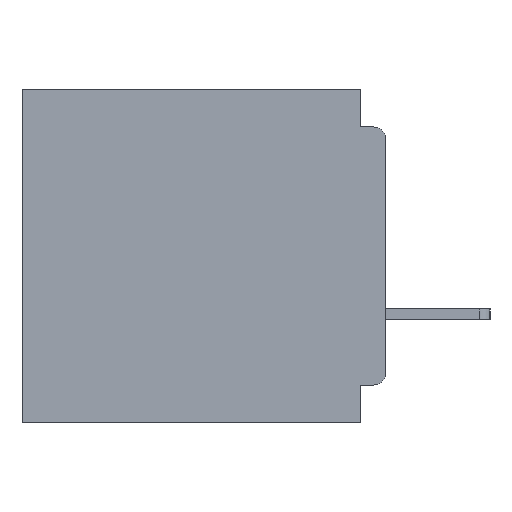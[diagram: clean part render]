
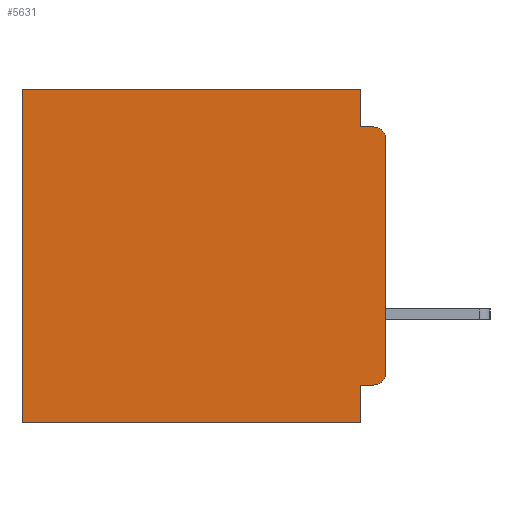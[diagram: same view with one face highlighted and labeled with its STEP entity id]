
A CAD part, left-side view. The second image highlights one B-rep face of the part: STEP entity #5631.
In plain terms, the highlighted planar face has unit normal (-1, 0, 0).
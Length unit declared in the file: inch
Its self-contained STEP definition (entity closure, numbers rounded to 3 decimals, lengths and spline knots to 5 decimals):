
#741 = EDGE_CURVE ( 'NONE', #38805, #25974, #11885, .T. ) ;
#1370 = DIRECTION ( 'NONE',  ( 0., 1., 0. ) ) ;
#1485 = CARTESIAN_POINT ( 'NONE',  ( 0.3, 0.031, -0.4 ) ) ;
#1677 = DIRECTION ( 'NONE',  ( 0., 0., -1. ) ) ;
#1824 = ORIENTED_EDGE ( 'NONE', *, *, #9214, .F. ) ;
#2013 = EDGE_CURVE ( 'NONE', #36168, #10395, #43363, .T. ) ;
#3082 = ORIENTED_EDGE ( 'NONE', *, *, #47708, .F. ) ;
#3362 = CARTESIAN_POINT ( 'NONE',  ( 0.3, 0.437, -0.4 ) ) ;
#3522 = VERTEX_POINT ( 'NONE', #3362 ) ;
#3754 = ORIENTED_EDGE ( 'NONE', *, *, #39988, .F. ) ;
#3835 = VERTEX_POINT ( 'NONE', #34441 ) ;
#4803 = LINE ( 'NONE', #1485, #13261 ) ;
#4859 = CARTESIAN_POINT ( 'NONE',  ( 0.3, 0.015, -0.06 ) ) ;
#5529 = CARTESIAN_POINT ( 'NONE',  ( 0.3, 0., -0.045 ) ) ;
#5631 = ADVANCED_FACE ( 'NONE', ( #22482 ), #20416, .F. ) ;
#7128 = AXIS2_PLACEMENT_3D ( 'NONE', #24564, #53194, #28710 ) ;
#7584 = ORIENTED_EDGE ( 'NONE', *, *, #47309, .F. ) ;
#7734 = EDGE_CURVE ( 'NONE', #50277, #3522, #35252, .T. ) ;
#9214 = EDGE_CURVE ( 'NONE', #19254, #3522, #44039, .T. ) ;
#10395 = VERTEX_POINT ( 'NONE', #48416 ) ;
#11695 = VECTOR ( 'NONE', #14573, 39.37008 ) ;
#11885 = CIRCLE ( 'NONE', #27965, 0.015 ) ;
#13144 = CARTESIAN_POINT ( 'NONE',  ( 0.3, 0.031, 0. ) ) ;
#13261 = VECTOR ( 'NONE', #1677, 39.37008 ) ;
#14573 = DIRECTION ( 'NONE',  ( 0., 1., 0. ) ) ;
#14928 = DIRECTION ( 'NONE',  ( 0., 0., -1. ) ) ;
#15295 = VECTOR ( 'NONE', #1370, 39.37008 ) ;
#15351 = VECTOR ( 'NONE', #14928, 39.37008 ) ;
#16631 = CARTESIAN_POINT ( 'NONE',  ( 0.3, 0.437, -0.4 ) ) ;
#18126 = VECTOR ( 'NONE', #34469, 39.37008 ) ;
#18258 = DIRECTION ( 'NONE',  ( 0., 1., 0. ) ) ;
#18376 = DIRECTION ( 'NONE',  ( -1., 0., 0. ) ) ;
#19254 = VERTEX_POINT ( 'NONE', #21197 ) ;
#19961 = DIRECTION ( 'NONE',  ( 0., 0., -1. ) ) ;
#20126 = LINE ( 'NONE', #39297, #11695 ) ;
#20416 = PLANE ( 'NONE',  #7128 ) ;
#21197 = CARTESIAN_POINT ( 'NONE',  ( 0.3, 0.031, -0.4 ) ) ;
#21206 = CARTESIAN_POINT ( 'NONE',  ( 0.3, 0., -0.4 ) ) ;
#22040 = CARTESIAN_POINT ( 'NONE',  ( 0.3, 0., 0. ) ) ;
#22136 = VECTOR ( 'NONE', #18258, 39.37008 ) ;
#22482 = FACE_OUTER_BOUND ( 'NONE', #44814, .T. ) ;
#23851 = AXIS2_PLACEMENT_3D ( 'NONE', #43078, #18376, #47183 ) ;
#24564 = CARTESIAN_POINT ( 'NONE',  ( 0.3, 0., -0.4 ) ) ;
#25974 = VERTEX_POINT ( 'NONE', #37132 ) ;
#27457 = ORIENTED_EDGE ( 'NONE', *, *, #741, .T. ) ;
#27965 = AXIS2_PLACEMENT_3D ( 'NONE', #4859, #35061, #19961 ) ;
#28710 = DIRECTION ( 'NONE',  ( 0., 0., -1. ) ) ;
#29030 = CARTESIAN_POINT ( 'NONE',  ( 0.3, 0.437, 0. ) ) ;
#29109 = LINE ( 'NONE', #5529, #18126 ) ;
#29497 = DIRECTION ( 'NONE',  ( 0., 0., -1. ) ) ;
#32095 = VERTEX_POINT ( 'NONE', #13144 ) ;
#34432 = EDGE_CURVE ( 'NONE', #32095, #3835, #48195, .T. ) ;
#34441 = CARTESIAN_POINT ( 'NONE',  ( 0.3, 0.031, -0.045 ) ) ;
#34469 = DIRECTION ( 'NONE',  ( 0., -1., 0. ) ) ;
#34699 = CARTESIAN_POINT ( 'NONE',  ( 0.3, 0., -0.4 ) ) ;
#35061 = DIRECTION ( 'NONE',  ( -1., 0., 0. ) ) ;
#35252 = LINE ( 'NONE', #16631, #44849 ) ;
#35336 = CARTESIAN_POINT ( 'NONE',  ( 0.3, 0.031, 0. ) ) ;
#36168 = VERTEX_POINT ( 'NONE', #38331 ) ;
#36844 = EDGE_CURVE ( 'NONE', #32095, #50277, #38521, .T. ) ;
#37132 = CARTESIAN_POINT ( 'NONE',  ( 0.3, 0.015, -0.045 ) ) ;
#37508 = EDGE_CURVE ( 'NONE', #51547, #19254, #4803, .T. ) ;
#37561 = CARTESIAN_POINT ( 'NONE',  ( 0.3, 0.031, -0.355 ) ) ;
#38331 = CARTESIAN_POINT ( 'NONE',  ( 0.3, 0.015, -0.355 ) ) ;
#38521 = LINE ( 'NONE', #22040, #15295 ) ;
#38805 = VERTEX_POINT ( 'NONE', #47325 ) ;
#39297 = CARTESIAN_POINT ( 'NONE',  ( 0.3, 0., -0.355 ) ) ;
#39988 = EDGE_CURVE ( 'NONE', #3835, #25974, #29109, .T. ) ;
#41125 = ORIENTED_EDGE ( 'NONE', *, *, #7734, .T. ) ;
#41318 = DIRECTION ( 'NONE',  ( 0., 0., -1. ) ) ;
#41329 = ORIENTED_EDGE ( 'NONE', *, *, #36844, .T. ) ;
#42000 = LINE ( 'NONE', #21206, #51550 ) ;
#43078 = CARTESIAN_POINT ( 'NONE',  ( 0.3, 0.015, -0.34 ) ) ;
#43363 = CIRCLE ( 'NONE', #23851, 0.015 ) ;
#44039 = LINE ( 'NONE', #34699, #22136 ) ;
#44814 = EDGE_LOOP ( 'NONE', ( #3082, #27457, #3754, #49943, #41329, #41125, #1824, #48296, #7584, #46086 ) ) ;
#44849 = VECTOR ( 'NONE', #41318, 39.37008 ) ;
#46086 = ORIENTED_EDGE ( 'NONE', *, *, #2013, .T. ) ;
#47183 = DIRECTION ( 'NONE',  ( 0., 0., -1. ) ) ;
#47309 = EDGE_CURVE ( 'NONE', #36168, #51547, #20126, .T. ) ;
#47325 = CARTESIAN_POINT ( 'NONE',  ( 0.3, 0., -0.06 ) ) ;
#47708 = EDGE_CURVE ( 'NONE', #38805, #10395, #42000, .T. ) ;
#48195 = LINE ( 'NONE', #35336, #15351 ) ;
#48296 = ORIENTED_EDGE ( 'NONE', *, *, #37508, .F. ) ;
#48416 = CARTESIAN_POINT ( 'NONE',  ( 0.3, 0., -0.34 ) ) ;
#49943 = ORIENTED_EDGE ( 'NONE', *, *, #34432, .F. ) ;
#50277 = VERTEX_POINT ( 'NONE', #29030 ) ;
#51547 = VERTEX_POINT ( 'NONE', #37561 ) ;
#51550 = VECTOR ( 'NONE', #29497, 39.37008 ) ;
#53194 = DIRECTION ( 'NONE',  ( 1., 0., 0. ) ) ;
